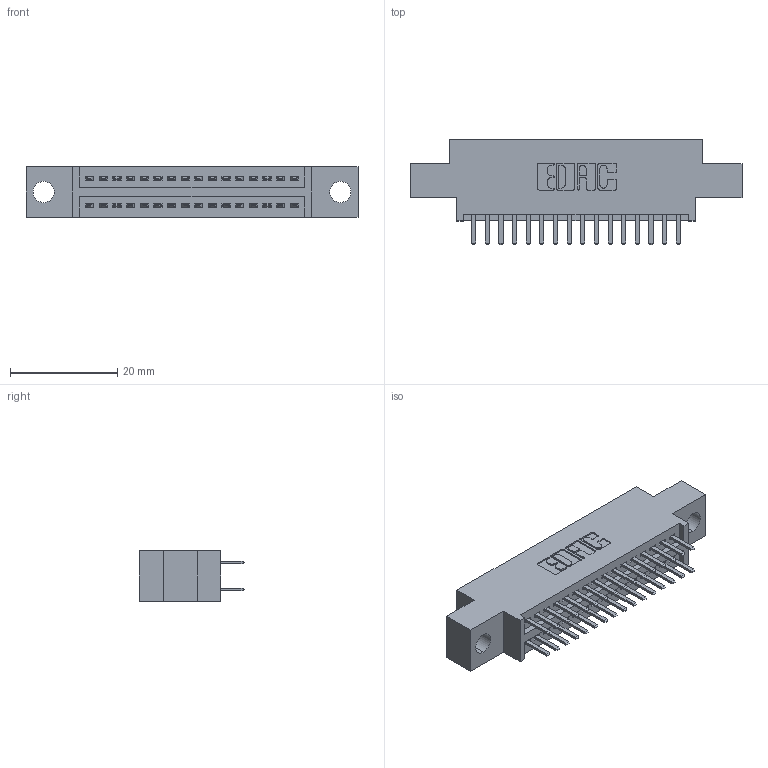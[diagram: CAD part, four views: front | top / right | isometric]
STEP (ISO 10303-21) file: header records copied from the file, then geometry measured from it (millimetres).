
FILE_DESCRIPTION (( 'STEP AP203' ), '1' );
FILE_NAME ('345-032-520-804.STEP', '2021-05-19T23:37:31', ( '' ), ( '' ), 'SwSTEP 2.0', 'SolidWorks 2020', '' );
FILE_SCHEMA (( 'CONFIG_CONTROL_DESIGN' ));
Length unit declared in the file: inch
Products named in the file (3): 345 Part_0.170 Offset - 0.156 Dia-TI; 345-032-520-804; 345-292-001_345-293-120
Assembly tree (33 placements, depth 2):
  345-032-520-804
    345 Part_0.170 Offset - 0.156 Dia-TI
    345-292-001_345-293-120  x32
Bounding box: 61.85 x 19.68 x 9.4 mm (x, y, z)
Volume: 5533.3 mm3; surface area: 7640.8 mm2
Topology: 33 solids, 33 shells, 1872 faces, 5413 edges, 3522 vertices
Faces by surface type: plane 1218, cylinder 654
Entity records: 16719 total; most frequent: CARTESIAN_POINT 2846, ORIENTED_EDGE 2766, DIRECTION 2527, EDGE_CURVE 1383, VECTOR 1183, LINE 1183, VERTEX_POINT 918, AXIS2_PLACEMENT_3D 672
